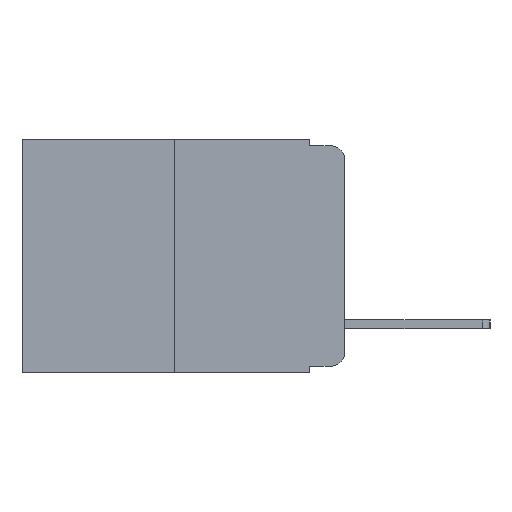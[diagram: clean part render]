
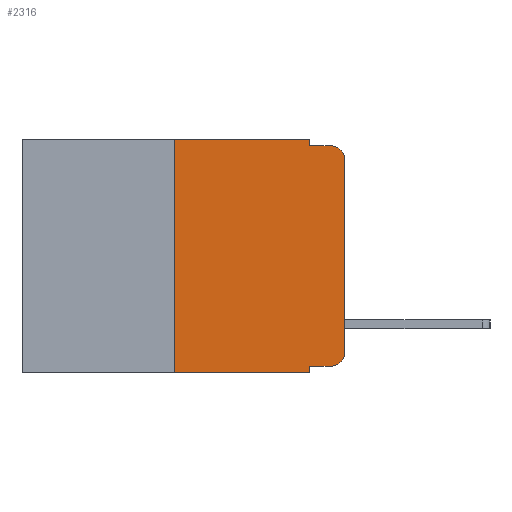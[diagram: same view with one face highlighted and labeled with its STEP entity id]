
A CAD part, left-side view. The second image highlights one B-rep face of the part: STEP entity #2316.
In plain terms, the highlighted planar face has unit normal (-1, 0, 0).
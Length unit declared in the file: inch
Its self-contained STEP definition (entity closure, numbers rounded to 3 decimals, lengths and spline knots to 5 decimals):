
#35 = CARTESIAN_POINT ( 'NONE',  ( 0., 0.02, -0.01 ) ) ;
#230 = EDGE_CURVE ( 'NONE', #6087, #2561, #17755, .T. ) ;
#580 = CARTESIAN_POINT ( 'NONE',  ( 0., 0.02, -0.333 ) ) ;
#975 = VERTEX_POINT ( 'NONE', #9504 ) ;
#1398 = CARTESIAN_POINT ( 'NONE',  ( 0., 0.473, 0. ) ) ;
#1498 = CARTESIAN_POINT ( 'NONE',  ( 0., 0.051, -0.333 ) ) ;
#2039 = VERTEX_POINT ( 'NONE', #14686 ) ;
#2070 = ORIENTED_EDGE ( 'NONE', *, *, #11584, .F. ) ;
#2283 = CIRCLE ( 'NONE', #9594, 0.02 ) ;
#2316 = ADVANCED_FACE ( 'NONE', ( #5514 ), #6906, .F. ) ;
#2339 = CARTESIAN_POINT ( 'NONE',  ( 0., 0.02, -0.03 ) ) ;
#2360 = CARTESIAN_POINT ( 'NONE',  ( 0., 0.473, -0.343 ) ) ;
#2373 = LINE ( 'NONE', #12538, #6554 ) ;
#2561 = VERTEX_POINT ( 'NONE', #580 ) ;
#2595 = CIRCLE ( 'NONE', #10281, 0.02 ) ;
#2783 = EDGE_LOOP ( 'NONE', ( #4941, #9106, #12756, #2070, #17149, #14010, #7123, #10866, #14834, #4288 ) ) ;
#3047 = DIRECTION ( 'NONE',  ( 0., 0., -1. ) ) ;
#3104 = DIRECTION ( 'NONE',  ( 0., 0., -1. ) ) ;
#3145 = EDGE_CURVE ( 'NONE', #6087, #15276, #3971, .T. ) ;
#3201 = CARTESIAN_POINT ( 'NONE',  ( 0., 0.051, -0.343 ) ) ;
#3206 = CARTESIAN_POINT ( 'NONE',  ( 0., 0.051, 0. ) ) ;
#3510 = VECTOR ( 'NONE', #14563, 39.37008 ) ;
#3768 = DIRECTION ( 'NONE',  ( 0., 0., -1. ) ) ;
#3793 = DIRECTION ( 'NONE',  ( 0., -1., 0. ) ) ;
#3863 = DIRECTION ( 'NONE',  ( -1., 0., 0. ) ) ;
#3971 = LINE ( 'NONE', #11487, #14534 ) ;
#4288 = ORIENTED_EDGE ( 'NONE', *, *, #17280, .T. ) ;
#4809 = VECTOR ( 'NONE', #16634, 39.37008 ) ;
#4939 = CARTESIAN_POINT ( 'NONE',  ( 0., 0.051, -0.01 ) ) ;
#4941 = ORIENTED_EDGE ( 'NONE', *, *, #15136, .T. ) ;
#5028 = VECTOR ( 'NONE', #3793, 39.37008 ) ;
#5448 = VERTEX_POINT ( 'NONE', #3206 ) ;
#5456 = LINE ( 'NONE', #2360, #5028 ) ;
#5514 = FACE_OUTER_BOUND ( 'NONE', #2783, .T. ) ;
#5715 = EDGE_CURVE ( 'NONE', #7401, #15276, #5456, .T. ) ;
#5849 = VECTOR ( 'NONE', #6977, 39.37008 ) ;
#5976 = EDGE_CURVE ( 'NONE', #10743, #5448, #8513, .T. ) ;
#6087 = VERTEX_POINT ( 'NONE', #12897 ) ;
#6378 = VECTOR ( 'NONE', #11004, 39.37008 ) ;
#6554 = VECTOR ( 'NONE', #8425, 39.37008 ) ;
#6771 = LINE ( 'NONE', #4939, #3510 ) ;
#6906 = PLANE ( 'NONE',  #8011 ) ;
#6977 = DIRECTION ( 'NONE',  ( 0., 0., 1. ) ) ;
#7123 = ORIENTED_EDGE ( 'NONE', *, *, #5715, .T. ) ;
#7348 = VECTOR ( 'NONE', #7643, 39.37008 ) ;
#7401 = VERTEX_POINT ( 'NONE', #12100 ) ;
#7643 = DIRECTION ( 'NONE',  ( 0., -1., 0. ) ) ;
#7843 = CARTESIAN_POINT ( 'NONE',  ( 0., 0., -0.03 ) ) ;
#8011 = AXIS2_PLACEMENT_3D ( 'NONE', #12260, #15455, #3047 ) ;
#8425 = DIRECTION ( 'NONE',  ( 0., 0., 1. ) ) ;
#8513 = LINE ( 'NONE', #1398, #4809 ) ;
#8773 = EDGE_CURVE ( 'NONE', #7401, #10743, #2373, .T. ) ;
#9106 = ORIENTED_EDGE ( 'NONE', *, *, #14259, .T. ) ;
#9504 = CARTESIAN_POINT ( 'NONE',  ( 0., 0., -0.313 ) ) ;
#9568 = CARTESIAN_POINT ( 'NONE',  ( 0., 0.051, 0. ) ) ;
#9594 = AXIS2_PLACEMENT_3D ( 'NONE', #12200, #3863, #13549 ) ;
#9938 = VERTEX_POINT ( 'NONE', #35 ) ;
#10030 = LINE ( 'NONE', #12451, #5849 ) ;
#10281 = AXIS2_PLACEMENT_3D ( 'NONE', #2339, #12125, #3768 ) ;
#10743 = VERTEX_POINT ( 'NONE', #13298 ) ;
#10866 = ORIENTED_EDGE ( 'NONE', *, *, #3145, .F. ) ;
#11004 = DIRECTION ( 'NONE',  ( 0., 0., -1. ) ) ;
#11487 = CARTESIAN_POINT ( 'NONE',  ( 0., 0.051, 0. ) ) ;
#11584 = EDGE_CURVE ( 'NONE', #5448, #2039, #17271, .T. ) ;
#12100 = CARTESIAN_POINT ( 'NONE',  ( 0., 0.25, -0.343 ) ) ;
#12125 = DIRECTION ( 'NONE',  ( -1., 0., 0. ) ) ;
#12200 = CARTESIAN_POINT ( 'NONE',  ( 0., 0.02, -0.313 ) ) ;
#12260 = CARTESIAN_POINT ( 'NONE',  ( 0., 0.473, 0. ) ) ;
#12451 = CARTESIAN_POINT ( 'NONE',  ( 0., 0., 0. ) ) ;
#12471 = EDGE_CURVE ( 'NONE', #2039, #9938, #6771, .T. ) ;
#12538 = CARTESIAN_POINT ( 'NONE',  ( 0., 0.25, 0. ) ) ;
#12756 = ORIENTED_EDGE ( 'NONE', *, *, #12471, .F. ) ;
#12897 = CARTESIAN_POINT ( 'NONE',  ( 0., 0.051, -0.333 ) ) ;
#13233 = VERTEX_POINT ( 'NONE', #7843 ) ;
#13298 = CARTESIAN_POINT ( 'NONE',  ( 0., 0.25, 0. ) ) ;
#13549 = DIRECTION ( 'NONE',  ( 0., 0., -1. ) ) ;
#14010 = ORIENTED_EDGE ( 'NONE', *, *, #8773, .F. ) ;
#14259 = EDGE_CURVE ( 'NONE', #13233, #9938, #2595, .T. ) ;
#14534 = VECTOR ( 'NONE', #3104, 39.37008 ) ;
#14563 = DIRECTION ( 'NONE',  ( 0., -1., 0. ) ) ;
#14686 = CARTESIAN_POINT ( 'NONE',  ( 0., 0.051, -0.01 ) ) ;
#14834 = ORIENTED_EDGE ( 'NONE', *, *, #230, .T. ) ;
#15136 = EDGE_CURVE ( 'NONE', #975, #13233, #10030, .T. ) ;
#15276 = VERTEX_POINT ( 'NONE', #3201 ) ;
#15455 = DIRECTION ( 'NONE',  ( 1., 0., 0. ) ) ;
#16634 = DIRECTION ( 'NONE',  ( 0., -1., 0. ) ) ;
#17149 = ORIENTED_EDGE ( 'NONE', *, *, #5976, .F. ) ;
#17271 = LINE ( 'NONE', #9568, #6378 ) ;
#17280 = EDGE_CURVE ( 'NONE', #2561, #975, #2283, .T. ) ;
#17755 = LINE ( 'NONE', #1498, #7348 ) ;
